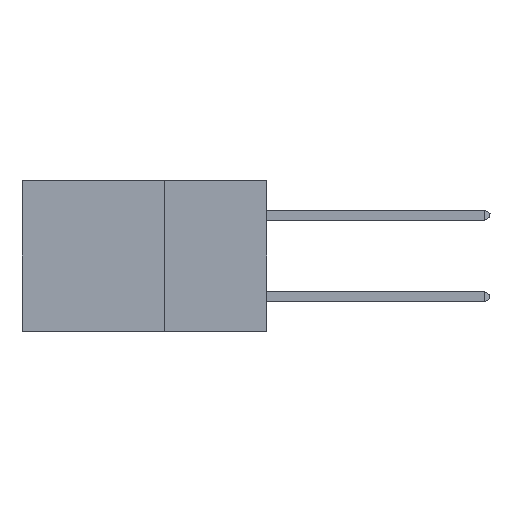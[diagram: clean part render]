
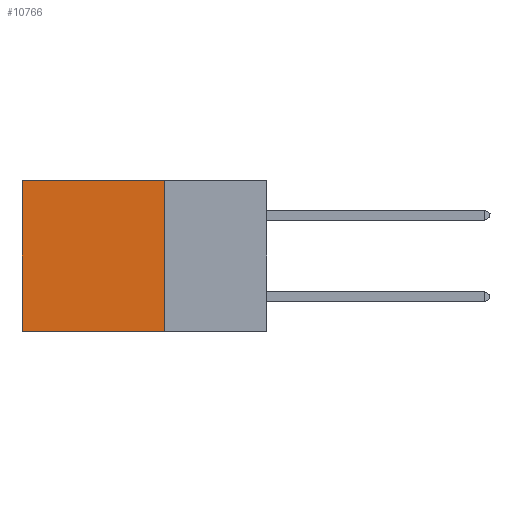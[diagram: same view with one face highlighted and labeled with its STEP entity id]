
A CAD part, left-side view. The second image highlights one B-rep face of the part: STEP entity #10766.
In plain terms, the highlighted planar face has unit normal (-1, 0, 0).
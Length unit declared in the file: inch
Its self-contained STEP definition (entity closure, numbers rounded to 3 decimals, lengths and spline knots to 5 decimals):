
#477 = LINE ( 'NONE', #6867, #16423 ) ;
#1100 = VECTOR ( 'NONE', #16625, 39.37008 ) ;
#3041 = EDGE_LOOP ( 'NONE', ( #15063, #3485, #14743, #9645 ) ) ;
#3390 = DIRECTION ( 'NONE',  ( 1., 0., 0. ) ) ;
#3485 = ORIENTED_EDGE ( 'NONE', *, *, #14629, .F. ) ;
#3920 = EDGE_CURVE ( 'NONE', #15198, #14773, #6473, .T. ) ;
#6473 = LINE ( 'NONE', #16489, #7935 ) ;
#6484 = DIRECTION ( 'NONE',  ( 0., 0., -1. ) ) ;
#6867 = CARTESIAN_POINT ( 'NONE',  ( 0.2875, 0.6, 0. ) ) ;
#7657 = FACE_OUTER_BOUND ( 'NONE', #3041, .T. ) ;
#7935 = VECTOR ( 'NONE', #19608, 39.37008 ) ;
#8200 = EDGE_CURVE ( 'NONE', #14773, #18776, #477, .T. ) ;
#8550 = DIRECTION ( 'NONE',  ( 0., 0., -1. ) ) ;
#8678 = CARTESIAN_POINT ( 'NONE',  ( 0.2875, 0.6, -0.37 ) ) ;
#8970 = DIRECTION ( 'NONE',  ( 0., 0., -1. ) ) ;
#9645 = ORIENTED_EDGE ( 'NONE', *, *, #3920, .T. ) ;
#10766 = ADVANCED_FACE ( 'NONE', ( #7657 ), #11786, .F. ) ;
#11129 = VERTEX_POINT ( 'NONE', #19183 ) ;
#11444 = VECTOR ( 'NONE', #8970, 39.37008 ) ;
#11783 = CARTESIAN_POINT ( 'NONE',  ( 0.2875, 0.25, 0. ) ) ;
#11786 = PLANE ( 'NONE',  #15740 ) ;
#11918 = LINE ( 'NONE', #15287, #11444 ) ;
#13843 = CARTESIAN_POINT ( 'NONE',  ( 0.2875, 0.6, 0. ) ) ;
#14629 = EDGE_CURVE ( 'NONE', #11129, #18776, #17995, .T. ) ;
#14743 = ORIENTED_EDGE ( 'NONE', *, *, #16044, .F. ) ;
#14773 = VERTEX_POINT ( 'NONE', #13843 ) ;
#15063 = ORIENTED_EDGE ( 'NONE', *, *, #8200, .T. ) ;
#15178 = CARTESIAN_POINT ( 'NONE',  ( 0.2875, 0.25, 0. ) ) ;
#15198 = VERTEX_POINT ( 'NONE', #11783 ) ;
#15287 = CARTESIAN_POINT ( 'NONE',  ( 0.2875, 0.25, 0. ) ) ;
#15740 = AXIS2_PLACEMENT_3D ( 'NONE', #15178, #3390, #6484 ) ;
#16044 = EDGE_CURVE ( 'NONE', #15198, #11129, #11918, .T. ) ;
#16423 = VECTOR ( 'NONE', #8550, 39.37008 ) ;
#16489 = CARTESIAN_POINT ( 'NONE',  ( 0.2875, 0.25, 0. ) ) ;
#16625 = DIRECTION ( 'NONE',  ( 0., 1., 0. ) ) ;
#17995 = LINE ( 'NONE', #18230, #1100 ) ;
#18230 = CARTESIAN_POINT ( 'NONE',  ( 0.2875, 0.25, -0.37 ) ) ;
#18776 = VERTEX_POINT ( 'NONE', #8678 ) ;
#19183 = CARTESIAN_POINT ( 'NONE',  ( 0.2875, 0.25, -0.37 ) ) ;
#19608 = DIRECTION ( 'NONE',  ( 0., 1., 0. ) ) ;
